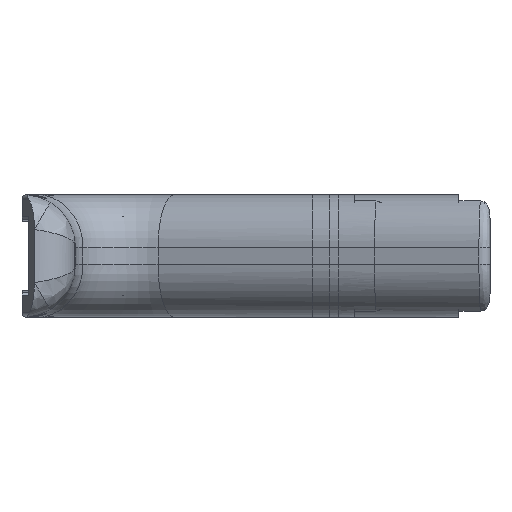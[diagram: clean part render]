
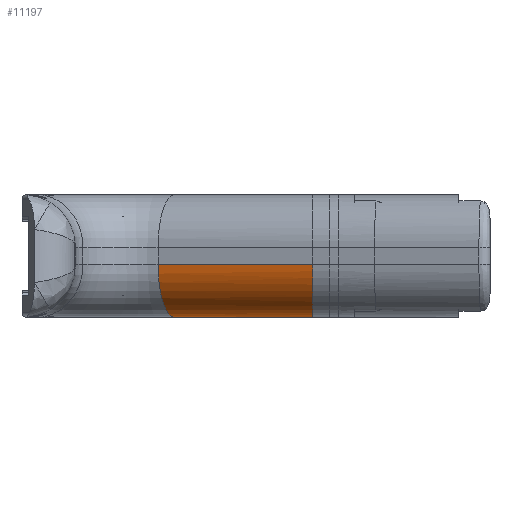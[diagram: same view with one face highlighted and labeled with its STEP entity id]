
A CAD part, left-side view. The second image highlights one B-rep face of the part: STEP entity #11197.
In plain terms, the highlighted cylindrical face has radius 12.5 mm (diameter 25 mm), a partial arc.
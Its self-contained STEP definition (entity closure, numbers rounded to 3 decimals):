
#269=ELLIPSE('',#11778,13.143,12.5);
#509=CYLINDRICAL_SURFACE('',#12081,12.5);
#955=FACE_OUTER_BOUND('',#1568,.T.);
#1568=EDGE_LOOP('',(#9260,#9261,#9262,#9263));
#1943=CIRCLE('',#11924,12.5);
#2275=LINE('',#16292,#3447);
#2789=LINE('',#19343,#3961);
#3447=VECTOR('',#13023,10.);
#3961=VECTOR('',#14419,10.);
#4592=VERTEX_POINT('',#16289);
#4593=VERTEX_POINT('',#16291);
#4796=VERTEX_POINT('',#17215);
#4946=VERTEX_POINT('',#18836);
#5759=EDGE_CURVE('',#4593,#4592,#2275,.T.);
#6045=EDGE_CURVE('',#4796,#4592,#269,.T.);
#6294=EDGE_CURVE('',#4946,#4593,#1943,.T.);
#6544=EDGE_CURVE('',#4796,#4946,#2789,.T.);
#9260=ORIENTED_EDGE('',*,*,#6045,.F.);
#9261=ORIENTED_EDGE('',*,*,#6544,.T.);
#9262=ORIENTED_EDGE('',*,*,#6294,.T.);
#9263=ORIENTED_EDGE('',*,*,#5759,.T.);
#11197=ADVANCED_FACE('',(#955),#509,.T.);
#11778=AXIS2_PLACEMENT_3D('',#17217,#13493,#13494);
#11924=AXIS2_PLACEMENT_3D('',#18837,#13901,#13902);
#12081=AXIS2_PLACEMENT_3D('',#19342,#14417,#14418);
#13023=DIRECTION('',(-0.309,-0.951,0.));
#13493=DIRECTION('center_axis',(0.,-1.,0.));
#13494=DIRECTION('ref_axis',(-1.,0.,0.));
#13901=DIRECTION('center_axis',(-0.309,-0.951,0.));
#13902=DIRECTION('ref_axis',(-0.951,0.309,0.));
#14417=DIRECTION('center_axis',(-0.309,-0.951,0.));
#14418=DIRECTION('ref_axis',(-0.672,0.219,-0.707));
#14419=DIRECTION('',(0.309,0.951,0.));
#16289=CARTESIAN_POINT('',(-64.797,-19.479,-34.));
#16291=CARTESIAN_POINT('',(-54.134,13.337,-34.));
#16292=CARTESIAN_POINT('',(-50.012,26.025,-34.));
#17215=CARTESIAN_POINT('',(-77.94,-19.479,-21.5));
#17217=CARTESIAN_POINT('Origin',(-64.797,-19.479,-21.5));
#18836=CARTESIAN_POINT('',(-66.022,17.2,-21.5));
#18837=CARTESIAN_POINT('Origin',(-54.134,13.337,-21.5));
#19342=CARTESIAN_POINT('Origin',(-50.012,26.025,-21.5));
#19343=CARTESIAN_POINT('',(-61.9,29.887,-21.5));
